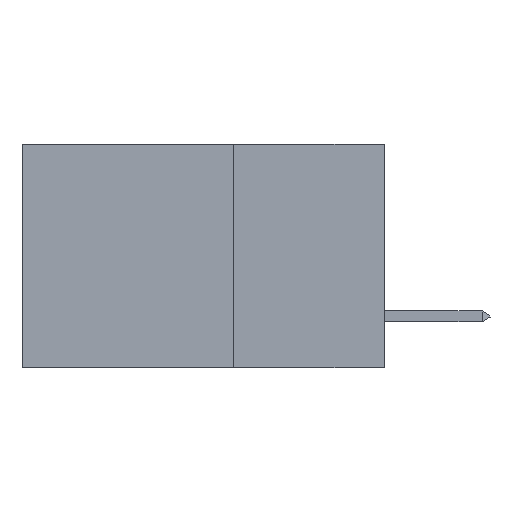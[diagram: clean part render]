
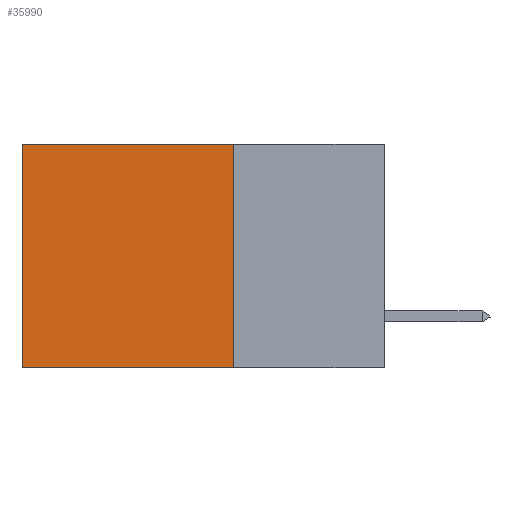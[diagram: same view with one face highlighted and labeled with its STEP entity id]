
A CAD part, left-side view. The second image highlights one B-rep face of the part: STEP entity #35990.
In plain terms, the highlighted planar face has unit normal (-1, 0, 0).
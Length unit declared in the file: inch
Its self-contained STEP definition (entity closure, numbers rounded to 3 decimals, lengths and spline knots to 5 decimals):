
#602 = CARTESIAN_POINT ( 'NONE',  ( 0.2875, 0.25, 0. ) ) ;
#1215 = DIRECTION ( 'NONE',  ( 0., 1., 0. ) ) ;
#1469 = LINE ( 'NONE', #602, #36020 ) ;
#2851 = CARTESIAN_POINT ( 'NONE',  ( 0.2875, 0.25, -0.37 ) ) ;
#3110 = LINE ( 'NONE', #35285, #8025 ) ;
#3199 = EDGE_CURVE ( 'NONE', #8402, #23215, #1469, .T. ) ;
#4053 = CARTESIAN_POINT ( 'NONE',  ( 0.2875, 0.6, 0. ) ) ;
#4355 = AXIS2_PLACEMENT_3D ( 'NONE', #19980, #16918, #19768 ) ;
#7512 = LINE ( 'NONE', #35480, #29178 ) ;
#8025 = VECTOR ( 'NONE', #21452, 39.37008 ) ;
#8402 = VERTEX_POINT ( 'NONE', #18136 ) ;
#10227 = ORIENTED_EDGE ( 'NONE', *, *, #32899, .F. ) ;
#12669 = CARTESIAN_POINT ( 'NONE',  ( 0.2875, 0.6, -0.37 ) ) ;
#13458 = VECTOR ( 'NONE', #1215, 39.37008 ) ;
#15243 = VERTEX_POINT ( 'NONE', #12669 ) ;
#16918 = DIRECTION ( 'NONE',  ( 1., 0., 0. ) ) ;
#18136 = CARTESIAN_POINT ( 'NONE',  ( 0.2875, 0.25, 0. ) ) ;
#18916 = ORIENTED_EDGE ( 'NONE', *, *, #3199, .F. ) ;
#19230 = LINE ( 'NONE', #32963, #13458 ) ;
#19768 = DIRECTION ( 'NONE',  ( 0., 0., -1. ) ) ;
#19980 = CARTESIAN_POINT ( 'NONE',  ( 0.2875, 0.25, 0. ) ) ;
#20062 = FACE_OUTER_BOUND ( 'NONE', #36301, .T. ) ;
#21452 = DIRECTION ( 'NONE',  ( 0., 0., -1. ) ) ;
#21940 = ORIENTED_EDGE ( 'NONE', *, *, #25640, .T. ) ;
#22852 = PLANE ( 'NONE',  #4355 ) ;
#23215 = VERTEX_POINT ( 'NONE', #2851 ) ;
#24015 = DIRECTION ( 'NONE',  ( 0., 1., 0. ) ) ;
#24220 = DIRECTION ( 'NONE',  ( 0., 0., -1. ) ) ;
#25640 = EDGE_CURVE ( 'NONE', #8402, #28945, #19230, .T. ) ;
#26752 = EDGE_CURVE ( 'NONE', #28945, #15243, #3110, .T. ) ;
#28945 = VERTEX_POINT ( 'NONE', #4053 ) ;
#29178 = VECTOR ( 'NONE', #24015, 39.37008 ) ;
#31258 = ORIENTED_EDGE ( 'NONE', *, *, #26752, .T. ) ;
#32899 = EDGE_CURVE ( 'NONE', #23215, #15243, #7512, .T. ) ;
#32963 = CARTESIAN_POINT ( 'NONE',  ( 0.2875, 0.25, 0. ) ) ;
#35285 = CARTESIAN_POINT ( 'NONE',  ( 0.2875, 0.6, 0. ) ) ;
#35480 = CARTESIAN_POINT ( 'NONE',  ( 0.2875, 0.25, -0.37 ) ) ;
#35990 = ADVANCED_FACE ( 'NONE', ( #20062 ), #22852, .F. ) ;
#36020 = VECTOR ( 'NONE', #24220, 39.37008 ) ;
#36301 = EDGE_LOOP ( 'NONE', ( #31258, #10227, #18916, #21940 ) ) ;
